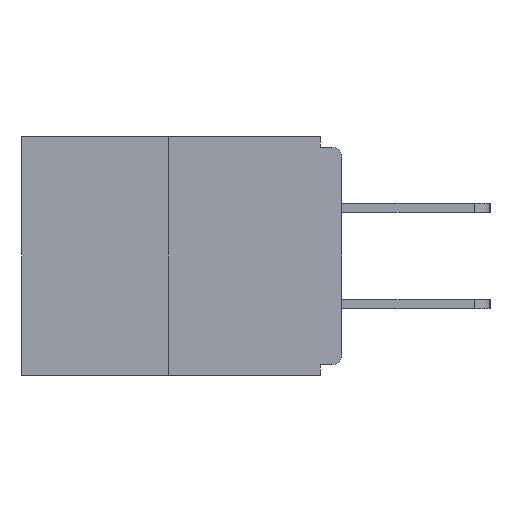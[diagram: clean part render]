
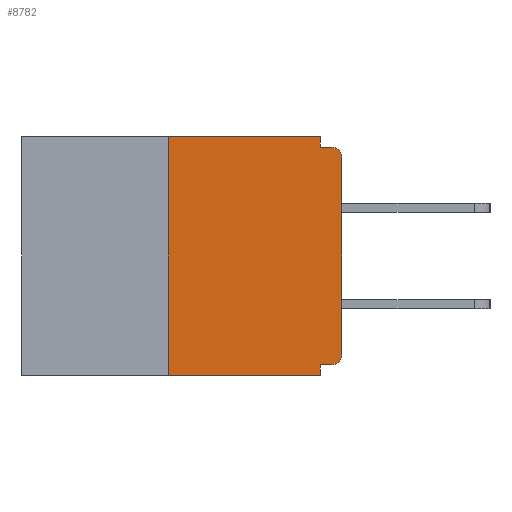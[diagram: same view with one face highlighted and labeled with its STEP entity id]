
A CAD part, left-side view. The second image highlights one B-rep face of the part: STEP entity #8782.
In plain terms, the highlighted planar face has unit normal (-1, 0, 0).
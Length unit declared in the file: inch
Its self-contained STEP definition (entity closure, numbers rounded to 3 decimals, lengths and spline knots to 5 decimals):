
#141 = EDGE_CURVE ( 'NONE', #12095, #17019, #12966, .T. ) ;
#216 = CARTESIAN_POINT ( 'NONE',  ( 0., 0.031, 0. ) ) ;
#821 = VECTOR ( 'NONE', #9960, 39.37008 ) ;
#1474 = EDGE_CURVE ( 'NONE', #21570, #12095, #11579, .T. ) ;
#1546 = DIRECTION ( 'NONE',  ( 1., 0., 0. ) ) ;
#1579 = VECTOR ( 'NONE', #19641, 39.37008 ) ;
#1876 = CARTESIAN_POINT ( 'NONE',  ( 0., 0.031, 0. ) ) ;
#2181 = CARTESIAN_POINT ( 'NONE',  ( 0., 0.015, -0.015 ) ) ;
#2414 = AXIS2_PLACEMENT_3D ( 'NONE', #14579, #4638, #17931 ) ;
#3114 = EDGE_CURVE ( 'NONE', #21570, #7497, #14806, .T. ) ;
#3163 = VERTEX_POINT ( 'NONE', #19927 ) ;
#3403 = LINE ( 'NONE', #21026, #1579 ) ;
#3645 = CARTESIAN_POINT ( 'NONE',  ( 0., 0.25, 0. ) ) ;
#3704 = EDGE_CURVE ( 'NONE', #7497, #3163, #4895, .T. ) ;
#3834 = CARTESIAN_POINT ( 'NONE',  ( 0., 0.015, -0.328 ) ) ;
#4638 = DIRECTION ( 'NONE',  ( -1., 0., 0. ) ) ;
#4894 = CARTESIAN_POINT ( 'NONE',  ( 0., 0., -0.328 ) ) ;
#4895 = LINE ( 'NONE', #9494, #6447 ) ;
#4958 = ORIENTED_EDGE ( 'NONE', *, *, #8685, .T. ) ;
#5466 = ORIENTED_EDGE ( 'NONE', *, *, #13876, .F. ) ;
#5502 = DIRECTION ( 'NONE',  ( 0., -1., 0. ) ) ;
#6230 = EDGE_CURVE ( 'NONE', #18787, #12924, #14386, .T. ) ;
#6447 = VECTOR ( 'NONE', #12873, 39.37008 ) ;
#6549 = CARTESIAN_POINT ( 'NONE',  ( 0., 0.46, 0. ) ) ;
#7025 = LINE ( 'NONE', #8608, #12262 ) ;
#7088 = DIRECTION ( 'NONE',  ( 0., 0., -1. ) ) ;
#7188 = EDGE_CURVE ( 'NONE', #12924, #8721, #10482, .T. ) ;
#7497 = VERTEX_POINT ( 'NONE', #13269 ) ;
#7634 = AXIS2_PLACEMENT_3D ( 'NONE', #20025, #8389, #20105 ) ;
#7639 = VERTEX_POINT ( 'NONE', #2181 ) ;
#8226 = CARTESIAN_POINT ( 'NONE',  ( 0., 0., 0. ) ) ;
#8389 = DIRECTION ( 'NONE',  ( -1., 0., 0. ) ) ;
#8608 = CARTESIAN_POINT ( 'NONE',  ( 0., 0., -0.015 ) ) ;
#8685 = EDGE_CURVE ( 'NONE', #9585, #3163, #3403, .T. ) ;
#8721 = VERTEX_POINT ( 'NONE', #17886 ) ;
#8782 = ADVANCED_FACE ( 'NONE', ( #11419 ), #14689, .F. ) ;
#9494 = CARTESIAN_POINT ( 'NONE',  ( 0., 0.031, -0.343 ) ) ;
#9585 = VERTEX_POINT ( 'NONE', #13283 ) ;
#9960 = DIRECTION ( 'NONE',  ( 0., 0., 1. ) ) ;
#10099 = CARTESIAN_POINT ( 'NONE',  ( 0., 0.25, 0. ) ) ;
#10482 = LINE ( 'NONE', #1876, #16946 ) ;
#11278 = CARTESIAN_POINT ( 'NONE',  ( 0., 0., -0.313 ) ) ;
#11419 = FACE_OUTER_BOUND ( 'NONE', #13009, .T. ) ;
#11579 = CIRCLE ( 'NONE', #7634, 0.015 ) ;
#12003 = ORIENTED_EDGE ( 'NONE', *, *, #1474, .T. ) ;
#12095 = VERTEX_POINT ( 'NONE', #11278 ) ;
#12262 = VECTOR ( 'NONE', #20256, 39.37008 ) ;
#12483 = EDGE_CURVE ( 'NONE', #9585, #18787, #12542, .T. ) ;
#12542 = LINE ( 'NONE', #10099, #821 ) ;
#12642 = AXIS2_PLACEMENT_3D ( 'NONE', #6549, #1546, #16402 ) ;
#12766 = ORIENTED_EDGE ( 'NONE', *, *, #3114, .F. ) ;
#12873 = DIRECTION ( 'NONE',  ( 0., 0., -1. ) ) ;
#12924 = VERTEX_POINT ( 'NONE', #216 ) ;
#12966 = LINE ( 'NONE', #8226, #17077 ) ;
#12974 = ORIENTED_EDGE ( 'NONE', *, *, #19478, .T. ) ;
#13009 = EDGE_LOOP ( 'NONE', ( #16355, #20087, #4958, #20755, #12766, #12003, #13643, #12974, #5466, #20321 ) ) ;
#13269 = CARTESIAN_POINT ( 'NONE',  ( 0., 0.031, -0.328 ) ) ;
#13283 = CARTESIAN_POINT ( 'NONE',  ( 0., 0.25, -0.343 ) ) ;
#13348 = DIRECTION ( 'NONE',  ( 0., 1., 0. ) ) ;
#13643 = ORIENTED_EDGE ( 'NONE', *, *, #141, .T. ) ;
#13876 = EDGE_CURVE ( 'NONE', #8721, #7639, #7025, .T. ) ;
#14386 = LINE ( 'NONE', #20260, #18279 ) ;
#14579 = CARTESIAN_POINT ( 'NONE',  ( 0., 0.015, -0.03 ) ) ;
#14689 = PLANE ( 'NONE',  #12642 ) ;
#14745 = CIRCLE ( 'NONE', #2414, 0.015 ) ;
#14806 = LINE ( 'NONE', #4894, #20527 ) ;
#16355 = ORIENTED_EDGE ( 'NONE', *, *, #6230, .F. ) ;
#16402 = DIRECTION ( 'NONE',  ( 0., 0., -1. ) ) ;
#16946 = VECTOR ( 'NONE', #7088, 39.37008 ) ;
#17019 = VERTEX_POINT ( 'NONE', #18192 ) ;
#17077 = VECTOR ( 'NONE', #19190, 39.37008 ) ;
#17886 = CARTESIAN_POINT ( 'NONE',  ( 0., 0.031, -0.015 ) ) ;
#17931 = DIRECTION ( 'NONE',  ( 0., 0., -1. ) ) ;
#18192 = CARTESIAN_POINT ( 'NONE',  ( 0., 0., -0.03 ) ) ;
#18279 = VECTOR ( 'NONE', #5502, 39.37008 ) ;
#18787 = VERTEX_POINT ( 'NONE', #3645 ) ;
#19190 = DIRECTION ( 'NONE',  ( 0., 0., 1. ) ) ;
#19478 = EDGE_CURVE ( 'NONE', #17019, #7639, #14745, .T. ) ;
#19641 = DIRECTION ( 'NONE',  ( 0., -1., 0. ) ) ;
#19927 = CARTESIAN_POINT ( 'NONE',  ( 0., 0.031, -0.343 ) ) ;
#20025 = CARTESIAN_POINT ( 'NONE',  ( 0., 0.015, -0.313 ) ) ;
#20087 = ORIENTED_EDGE ( 'NONE', *, *, #12483, .F. ) ;
#20105 = DIRECTION ( 'NONE',  ( 0., 0., -1. ) ) ;
#20256 = DIRECTION ( 'NONE',  ( 0., -1., 0. ) ) ;
#20260 = CARTESIAN_POINT ( 'NONE',  ( 0., 0.46, 0. ) ) ;
#20321 = ORIENTED_EDGE ( 'NONE', *, *, #7188, .F. ) ;
#20527 = VECTOR ( 'NONE', #13348, 39.37008 ) ;
#20755 = ORIENTED_EDGE ( 'NONE', *, *, #3704, .F. ) ;
#21026 = CARTESIAN_POINT ( 'NONE',  ( 0., 0.46, -0.343 ) ) ;
#21570 = VERTEX_POINT ( 'NONE', #3834 ) ;
